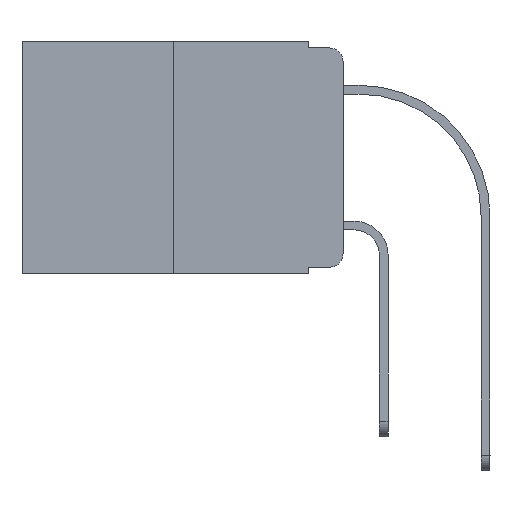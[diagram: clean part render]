
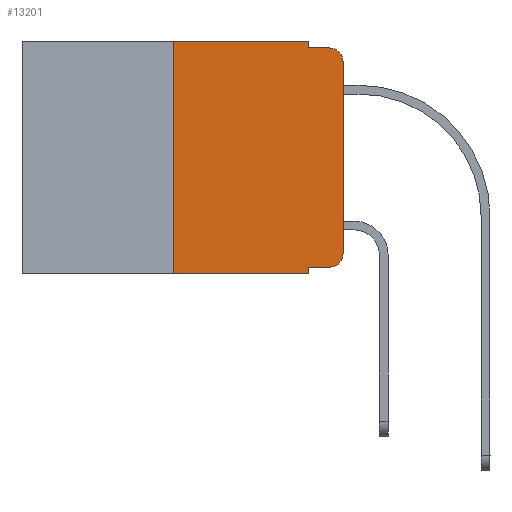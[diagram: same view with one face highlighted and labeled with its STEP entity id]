
A CAD part, left-side view. The second image highlights one B-rep face of the part: STEP entity #13201.
In plain terms, the highlighted planar face has unit normal (-1, 0, 0).
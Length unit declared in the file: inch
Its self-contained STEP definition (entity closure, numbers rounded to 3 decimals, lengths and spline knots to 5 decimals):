
#318 = CARTESIAN_POINT ( 'NONE',  ( 0., 0.02, -0.313 ) ) ;
#1104 = DIRECTION ( 'NONE',  ( 0., 0., 1. ) ) ;
#1308 = CARTESIAN_POINT ( 'NONE',  ( 0., 0.051, 0. ) ) ;
#1336 = ORIENTED_EDGE ( 'NONE', *, *, #12762, .T. ) ;
#1660 = CARTESIAN_POINT ( 'NONE',  ( 0., 0.473, 0. ) ) ;
#1721 = EDGE_CURVE ( 'NONE', #11557, #17044, #11392, .T. ) ;
#1819 = AXIS2_PLACEMENT_3D ( 'NONE', #9996, #4377, #9728 ) ;
#2386 = EDGE_LOOP ( 'NONE', ( #2977, #9193, #5115, #3241, #13284, #12651, #7137, #7253, #1336, #14110 ) ) ;
#2630 = EDGE_CURVE ( 'NONE', #11195, #8902, #12070, .T. ) ;
#2977 = ORIENTED_EDGE ( 'NONE', *, *, #10816, .T. ) ;
#3047 = LINE ( 'NONE', #1660, #8848 ) ;
#3241 = ORIENTED_EDGE ( 'NONE', *, *, #11795, .F. ) ;
#3317 = DIRECTION ( 'NONE',  ( 0., -1., 0. ) ) ;
#4115 = DIRECTION ( 'NONE',  ( -1., 0., 0. ) ) ;
#4138 = CARTESIAN_POINT ( 'NONE',  ( 0., 0.051, -0.01 ) ) ;
#4258 = AXIS2_PLACEMENT_3D ( 'NONE', #8508, #5962, #4738 ) ;
#4377 = DIRECTION ( 'NONE',  ( -1., 0., 0. ) ) ;
#4439 = CARTESIAN_POINT ( 'NONE',  ( 0., 0.473, -0.343 ) ) ;
#4593 = VECTOR ( 'NONE', #8563, 39.37008 ) ;
#4738 = DIRECTION ( 'NONE',  ( 0., 0., -1. ) ) ;
#5048 = CARTESIAN_POINT ( 'NONE',  ( 0., 0., 0. ) ) ;
#5115 = ORIENTED_EDGE ( 'NONE', *, *, #14603, .F. ) ;
#5272 = VERTEX_POINT ( 'NONE', #1308 ) ;
#5670 = DIRECTION ( 'NONE',  ( 0., 0., -1. ) ) ;
#5962 = DIRECTION ( 'NONE',  ( 1., 0., 0. ) ) ;
#5980 = CARTESIAN_POINT ( 'NONE',  ( 0., 0.051, -0.333 ) ) ;
#6135 = FACE_OUTER_BOUND ( 'NONE', #2386, .T. ) ;
#6366 = EDGE_CURVE ( 'NONE', #13903, #5272, #3047, .T. ) ;
#6446 = EDGE_CURVE ( 'NONE', #9160, #15867, #11061, .T. ) ;
#6538 = DIRECTION ( 'NONE',  ( 0., 0., -1. ) ) ;
#6625 = CARTESIAN_POINT ( 'NONE',  ( 0., 0.051, 0. ) ) ;
#6807 = VECTOR ( 'NONE', #16342, 39.37008 ) ;
#6924 = CARTESIAN_POINT ( 'NONE',  ( 0., 0., -0.313 ) ) ;
#7127 = LINE ( 'NONE', #5980, #7590 ) ;
#7137 = ORIENTED_EDGE ( 'NONE', *, *, #8210, .T. ) ;
#7253 = ORIENTED_EDGE ( 'NONE', *, *, #2630, .F. ) ;
#7453 = CARTESIAN_POINT ( 'NONE',  ( 0., 0.051, -0.01 ) ) ;
#7523 = CARTESIAN_POINT ( 'NONE',  ( 0., 0.02, -0.333 ) ) ;
#7550 = DIRECTION ( 'NONE',  ( 0., -1., 0. ) ) ;
#7590 = VECTOR ( 'NONE', #7550, 39.37008 ) ;
#8016 = CARTESIAN_POINT ( 'NONE',  ( 0., 0.051, -0.333 ) ) ;
#8210 = EDGE_CURVE ( 'NONE', #10272, #8902, #14032, .T. ) ;
#8508 = CARTESIAN_POINT ( 'NONE',  ( 0., 0.473, 0. ) ) ;
#8563 = DIRECTION ( 'NONE',  ( 0., -1., 0. ) ) ;
#8848 = VECTOR ( 'NONE', #3317, 39.37008 ) ;
#8902 = VERTEX_POINT ( 'NONE', #15752 ) ;
#9160 = VERTEX_POINT ( 'NONE', #16704 ) ;
#9193 = ORIENTED_EDGE ( 'NONE', *, *, #6446, .T. ) ;
#9252 = DIRECTION ( 'NONE',  ( 0., 0., 1. ) ) ;
#9450 = CARTESIAN_POINT ( 'NONE',  ( 0., 0.25, 0. ) ) ;
#9728 = DIRECTION ( 'NONE',  ( 0., 0., -1. ) ) ;
#9996 = CARTESIAN_POINT ( 'NONE',  ( 0., 0.02, -0.03 ) ) ;
#10096 = LINE ( 'NONE', #7453, #12610 ) ;
#10272 = VERTEX_POINT ( 'NONE', #10474 ) ;
#10474 = CARTESIAN_POINT ( 'NONE',  ( 0., 0.25, -0.343 ) ) ;
#10803 = VECTOR ( 'NONE', #6538, 39.37008 ) ;
#10816 = EDGE_CURVE ( 'NONE', #17044, #9160, #13150, .T. ) ;
#11061 = CIRCLE ( 'NONE', #1819, 0.02 ) ;
#11195 = VERTEX_POINT ( 'NONE', #8016 ) ;
#11234 = EDGE_CURVE ( 'NONE', #10272, #13903, #17256, .T. ) ;
#11392 = CIRCLE ( 'NONE', #16404, 0.02 ) ;
#11557 = VERTEX_POINT ( 'NONE', #7523 ) ;
#11795 = EDGE_CURVE ( 'NONE', #5272, #15652, #12119, .T. ) ;
#12070 = LINE ( 'NONE', #6625, #10803 ) ;
#12119 = LINE ( 'NONE', #14932, #6807 ) ;
#12226 = VECTOR ( 'NONE', #9252, 39.37008 ) ;
#12610 = VECTOR ( 'NONE', #16119, 39.37008 ) ;
#12651 = ORIENTED_EDGE ( 'NONE', *, *, #11234, .F. ) ;
#12762 = EDGE_CURVE ( 'NONE', #11195, #11557, #7127, .T. ) ;
#13150 = LINE ( 'NONE', #5048, #16268 ) ;
#13201 = ADVANCED_FACE ( 'NONE', ( #6135 ), #16778, .F. ) ;
#13284 = ORIENTED_EDGE ( 'NONE', *, *, #6366, .F. ) ;
#13401 = CARTESIAN_POINT ( 'NONE',  ( 0., 0.25, 0. ) ) ;
#13787 = CARTESIAN_POINT ( 'NONE',  ( 0., 0.02, -0.01 ) ) ;
#13903 = VERTEX_POINT ( 'NONE', #9450 ) ;
#14032 = LINE ( 'NONE', #4439, #4593 ) ;
#14110 = ORIENTED_EDGE ( 'NONE', *, *, #1721, .T. ) ;
#14603 = EDGE_CURVE ( 'NONE', #15652, #15867, #10096, .T. ) ;
#14932 = CARTESIAN_POINT ( 'NONE',  ( 0., 0.051, 0. ) ) ;
#15652 = VERTEX_POINT ( 'NONE', #4138 ) ;
#15752 = CARTESIAN_POINT ( 'NONE',  ( 0., 0.051, -0.343 ) ) ;
#15867 = VERTEX_POINT ( 'NONE', #13787 ) ;
#16119 = DIRECTION ( 'NONE',  ( 0., -1., 0. ) ) ;
#16268 = VECTOR ( 'NONE', #1104, 39.37008 ) ;
#16342 = DIRECTION ( 'NONE',  ( 0., 0., -1. ) ) ;
#16404 = AXIS2_PLACEMENT_3D ( 'NONE', #318, #4115, #5670 ) ;
#16704 = CARTESIAN_POINT ( 'NONE',  ( 0., 0., -0.03 ) ) ;
#16778 = PLANE ( 'NONE',  #4258 ) ;
#17044 = VERTEX_POINT ( 'NONE', #6924 ) ;
#17256 = LINE ( 'NONE', #13401, #12226 ) ;
